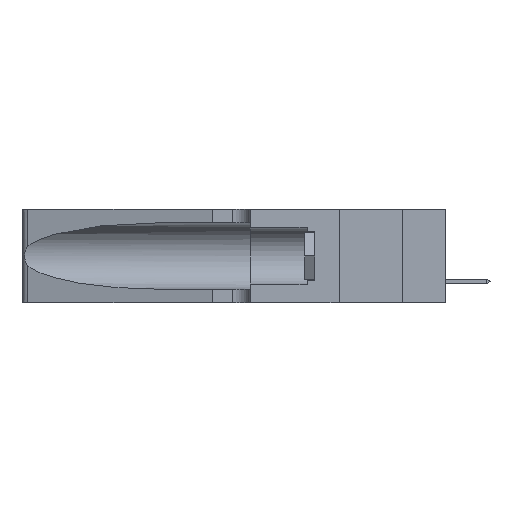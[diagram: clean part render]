
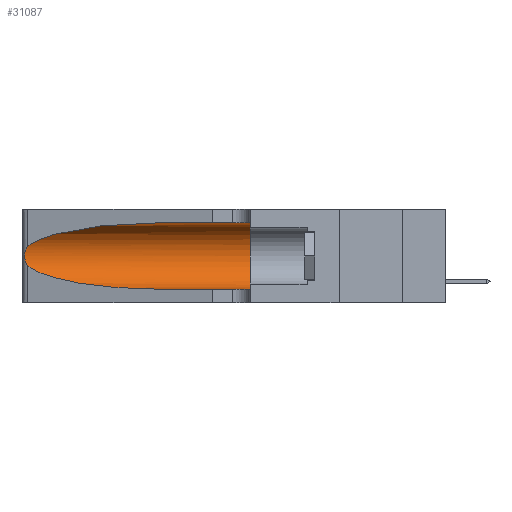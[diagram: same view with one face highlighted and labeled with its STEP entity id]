
A CAD part, left-side view. The second image highlights one B-rep face of the part: STEP entity #31087.
In plain terms, the highlighted cylindrical face has radius 3.308 mm (diameter 6.617 mm), a partial arc.
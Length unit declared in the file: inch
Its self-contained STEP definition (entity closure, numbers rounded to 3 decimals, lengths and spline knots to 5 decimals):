
#332 = CARTESIAN_POINT ( 'NONE',  ( 0.1305, 1.61858, 0.185 ) ) ;
#1263 = CARTESIAN_POINT ( 'NONE',  ( 0.25639, 1.23186, 0.15144 ) ) ;
#1638 = EDGE_CURVE ( 'NONE', #9961, #8539, #12076, .T. ) ;
#3467 = CARTESIAN_POINT ( 'NONE',  ( 0.25787, 1.23484, 0.2124 ) ) ;
#3695 = EDGE_LOOP ( 'NONE', ( #31768, #42355, #48792, #8931, #28030, #38627 ) ) ;
#4557 = CARTESIAN_POINT ( 'NONE',  ( 0.1305, 0.35, 0.05475 ) ) ;
#4838 = VERTEX_POINT ( 'NONE', #44945 ) ;
#4859 = CARTESIAN_POINT ( 'NONE',  ( 0.25789, 1.23486, 0.15765 ) ) ;
#5357 = CARTESIAN_POINT ( 'NONE',  ( 0.25555, 1.22993, 0.14849 ) ) ;
#5473 = CARTESIAN_POINT ( 'NONE',  ( 0.1305, 1.61858, 0.31525 ) ) ;
#6658 = CARTESIAN_POINT ( 'NONE',  ( 0.1305, 0.72297, 0.31525 ) ) ;
#8539 = VERTEX_POINT ( 'NONE', #4557 ) ;
#8931 = ORIENTED_EDGE ( 'NONE', *, *, #1638, .T. ) ;
#8993 = CARTESIAN_POINT ( 'NONE',  ( 0.26017, 1.23833, 0.17102 ) ) ;
#9961 = VERTEX_POINT ( 'NONE', #14686 ) ;
#10939 = CARTESIAN_POINT ( 'NONE',  ( 0.25487, 1.22718, 0.14631 ) ) ;
#12076 = LINE ( 'NONE', #24761, #21274 ) ;
#12163 = CARTESIAN_POINT ( 'NONE',  ( 0.25487, 1.22718, 0.14631 ) ) ;
#13078 = EDGE_CURVE ( 'NONE', #4838, #42879, #50728, .T. ) ;
#13174 = LINE ( 'NONE', #5473, #37612 ) ;
#13470 = AXIS2_PLACEMENT_3D ( 'NONE', #46873, #23308, #50304 ) ;
#14686 = CARTESIAN_POINT ( 'NONE',  ( 0.1305, 0.72297, 0.05475 ) ) ;
#16128 = CARTESIAN_POINT ( 'NONE',  ( 0.1305, 0.72297, 0.05475 ) ) ;
#16799 = CARTESIAN_POINT ( 'NONE',  ( 0.18966, 0.96281, 0.05475 ) ) ;
#17993 = FACE_OUTER_BOUND ( 'NONE', #3695, .T. ) ;
#18101 = CARTESIAN_POINT ( 'NONE',  ( 0.18966, 0.96281, 0.31525 ) ) ;
#19463 = CARTESIAN_POINT ( 'NONE',  ( 0.25555, 1.22994, 0.2215 ) ) ;
#20827 = CARTESIAN_POINT ( 'NONE',  ( 0.25487, 1.22718, 0.14631 ) ) ;
#21172 = VERTEX_POINT ( 'NONE', #46901 ) ;
#21274 = VECTOR ( 'NONE', #43496, 39.37008 ) ;
#22713 = CARTESIAN_POINT ( 'NONE',  ( 0.25854, 1.2359, 0.20912 ) ) ;
#22751 = EDGE_CURVE ( 'NONE', #26372, #21172, #13174, .T. ) ;
#23308 = DIRECTION ( 'NONE',  ( 0., 1., 0. ) ) ;
#24761 = CARTESIAN_POINT ( 'NONE',  ( 0.1305, 1.61858, 0.05475 ) ) ;
#24947 = CARTESIAN_POINT ( 'NONE',  ( 0.26075, 1.23896, 0.178 ) ) ;
#26372 = VERTEX_POINT ( 'NONE', #6658 ) ;
#27846 = CARTESIAN_POINT ( 'NONE',  ( 0.25487, 1.22718, 0.22369 ) ) ;
#28030 = ORIENTED_EDGE ( 'NONE', *, *, #30865, .F. ) ;
#29239 = AXIS2_PLACEMENT_3D ( 'NONE', #332, #43750, #35582 ) ;
#29636 = CIRCLE ( 'NONE', #13470, 0.13025 ) ;
#30865 = EDGE_CURVE ( 'NONE', #21172, #8539, #29636, .T. ) ;
#31087 = ADVANCED_FACE ( 'NONE', ( #17993 ), #35722, .F. ) ;
#31768 = ORIENTED_EDGE ( 'NONE', *, *, #45641, .T. ) ;
#31934 =( BOUNDED_CURVE ( )  B_SPLINE_CURVE ( 3, ( #34749, #18101, #46107, #27846 ),
 .UNSPECIFIED., .F., .F. ) 
 B_SPLINE_CURVE_WITH_KNOTS ( ( 4, 4 ),
 ( 1.5708, 2.84003 ),
 .UNSPECIFIED. ) 
 CURVE ( )  GEOMETRIC_REPRESENTATION_ITEM ( )  RATIONAL_B_SPLINE_CURVE ( ( 1., 0.87, 0.87, 1. ) ) 
 REPRESENTATION_ITEM ( '' )  );
#34496 = CARTESIAN_POINT ( 'NONE',  ( 0.26075, 1.23896, 0.19203 ) ) ;
#34749 = CARTESIAN_POINT ( 'NONE',  ( 0.1305, 0.72297, 0.31525 ) ) ;
#35582 = DIRECTION ( 'NONE',  ( 0., 0., -1. ) ) ;
#35722 = CYLINDRICAL_SURFACE ( 'NONE', #29239, 0.13025 ) ;
#37612 = VECTOR ( 'NONE', #40184, 39.37008 ) ;
#38593 = EDGE_CURVE ( 'NONE', #42879, #9961, #43174, .T. ) ;
#38627 = ORIENTED_EDGE ( 'NONE', *, *, #22751, .F. ) ;
#39642 = CARTESIAN_POINT ( 'NONE',  ( 0.2373, 1.15595, 0.08982 ) ) ;
#40184 = DIRECTION ( 'NONE',  ( 0., -1., 0. ) ) ;
#42355 = ORIENTED_EDGE ( 'NONE', *, *, #13078, .T. ) ;
#42879 = VERTEX_POINT ( 'NONE', #10939 ) ;
#43174 =( BOUNDED_CURVE ( )  B_SPLINE_CURVE ( 3, ( #12163, #39642, #16799, #16128 ),
 .UNSPECIFIED., .F., .T. ) 
 B_SPLINE_CURVE_WITH_KNOTS ( ( 4, 4 ),
 ( 3.44316, 4.71239 ),
 .UNSPECIFIED. ) 
 CURVE ( )  GEOMETRIC_REPRESENTATION_ITEM ( )  RATIONAL_B_SPLINE_CURVE ( ( 1., 0.87, 0.87, 1. ) ) 
 REPRESENTATION_ITEM ( '' )  );
#43496 = DIRECTION ( 'NONE',  ( 0., -1., 0. ) ) ;
#43750 = DIRECTION ( 'NONE',  ( 0., -1., 0. ) ) ;
#44945 = CARTESIAN_POINT ( 'NONE',  ( 0.25487, 1.22718, 0.22369 ) ) ;
#45641 = EDGE_CURVE ( 'NONE', #26372, #4838, #31934, .T. ) ;
#46107 = CARTESIAN_POINT ( 'NONE',  ( 0.2373, 1.15595, 0.28018 ) ) ;
#46113 = CARTESIAN_POINT ( 'NONE',  ( 0.25639, 1.23184, 0.21858 ) ) ;
#46873 = CARTESIAN_POINT ( 'NONE',  ( 0.1305, 0.35, 0.185 ) ) ;
#46901 = CARTESIAN_POINT ( 'NONE',  ( 0.1305, 0.35, 0.31525 ) ) ;
#48326 = CARTESIAN_POINT ( 'NONE',  ( 0.25856, 1.23593, 0.16098 ) ) ;
#48792 = ORIENTED_EDGE ( 'NONE', *, *, #38593, .T. ) ;
#50042 = CARTESIAN_POINT ( 'NONE',  ( 0.26018, 1.23835, 0.19895 ) ) ;
#50304 = DIRECTION ( 'NONE',  ( 0., 0., 1. ) ) ;
#50388 = CARTESIAN_POINT ( 'NONE',  ( 0.25487, 1.22718, 0.22369 ) ) ;
#50728 = B_SPLINE_CURVE_WITH_KNOTS ( 'NONE', 3,
 ( #50388, #19463, #46113, #3467, #22713, #50042, #34496, #24947, #8993, #48326, #4859, #1263, #5357, #20827 ),
 .UNSPECIFIED., .F., .F.,
 ( 4, 2, 2, 2, 2, 2, 4 ),
 ( 0., 0.00027, 0.00053, 0.00107, 0.0016, 0.00187, 0.00214 ),
 .UNSPECIFIED. ) ;
